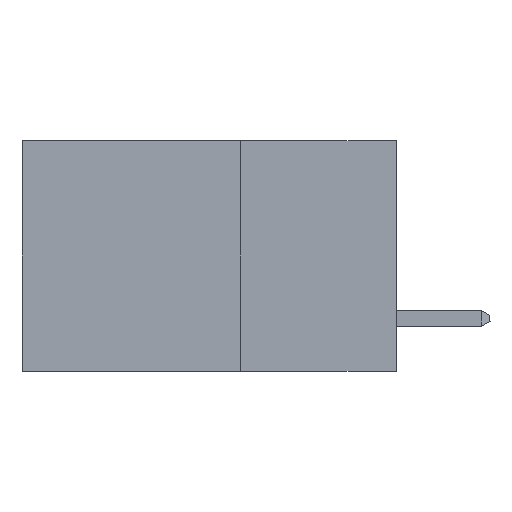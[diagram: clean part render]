
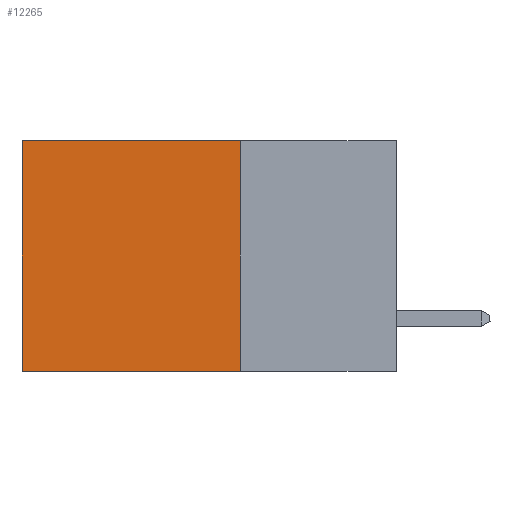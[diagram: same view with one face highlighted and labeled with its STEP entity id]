
A CAD part, left-side view. The second image highlights one B-rep face of the part: STEP entity #12265.
In plain terms, the highlighted planar face has unit normal (-1, 0, 0).
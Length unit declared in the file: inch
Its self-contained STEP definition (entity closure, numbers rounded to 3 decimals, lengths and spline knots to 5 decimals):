
#1314 = CARTESIAN_POINT ( 'NONE',  ( 0.298, 0.25, -0.37 ) ) ;
#1903 = VECTOR ( 'NONE', #5200, 39.37008 ) ;
#2294 = LINE ( 'NONE', #10504, #6072 ) ;
#2496 = VECTOR ( 'NONE', #14738, 39.37008 ) ;
#2888 = LINE ( 'NONE', #11260, #2496 ) ;
#3197 = ORIENTED_EDGE ( 'NONE', *, *, #7433, .F. ) ;
#3835 = DIRECTION ( 'NONE',  ( 1., 0., 0. ) ) ;
#4267 = ORIENTED_EDGE ( 'NONE', *, *, #6410, .T. ) ;
#5200 = DIRECTION ( 'NONE',  ( 0., 0., -1. ) ) ;
#5435 = CARTESIAN_POINT ( 'NONE',  ( 0.298, 0.6, 0. ) ) ;
#5701 = LINE ( 'NONE', #10752, #1903 ) ;
#6072 = VECTOR ( 'NONE', #12417, 39.37008 ) ;
#6164 = DIRECTION ( 'NONE',  ( 0., 1., 0. ) ) ;
#6410 = EDGE_CURVE ( 'NONE', #11763, #14839, #2294, .T. ) ;
#7433 = EDGE_CURVE ( 'NONE', #15279, #11608, #5701, .T. ) ;
#7614 = CARTESIAN_POINT ( 'NONE',  ( 0.298, 0.25, 0. ) ) ;
#9428 = CARTESIAN_POINT ( 'NONE',  ( 0.298, 0.25, 0. ) ) ;
#9562 = ORIENTED_EDGE ( 'NONE', *, *, #10904, .F. ) ;
#10504 = CARTESIAN_POINT ( 'NONE',  ( 0.298, 0.6, 0. ) ) ;
#10603 = LINE ( 'NONE', #12222, #13669 ) ;
#10654 = AXIS2_PLACEMENT_3D ( 'NONE', #7614, #3835, #12435 ) ;
#10752 = CARTESIAN_POINT ( 'NONE',  ( 0.298, 0.25, 0. ) ) ;
#10904 = EDGE_CURVE ( 'NONE', #11608, #14839, #10603, .T. ) ;
#11089 = ORIENTED_EDGE ( 'NONE', *, *, #12713, .T. ) ;
#11260 = CARTESIAN_POINT ( 'NONE',  ( 0.298, 0.25, 0. ) ) ;
#11272 = PLANE ( 'NONE',  #10654 ) ;
#11608 = VERTEX_POINT ( 'NONE', #1314 ) ;
#11763 = VERTEX_POINT ( 'NONE', #5435 ) ;
#12222 = CARTESIAN_POINT ( 'NONE',  ( 0.298, 0.25, -0.37 ) ) ;
#12265 = ADVANCED_FACE ( 'NONE', ( #13807 ), #11272, .F. ) ;
#12417 = DIRECTION ( 'NONE',  ( 0., 0., -1. ) ) ;
#12435 = DIRECTION ( 'NONE',  ( 0., 0., -1. ) ) ;
#12713 = EDGE_CURVE ( 'NONE', #15279, #11763, #2888, .T. ) ;
#13669 = VECTOR ( 'NONE', #6164, 39.37008 ) ;
#13807 = FACE_OUTER_BOUND ( 'NONE', #13974, .T. ) ;
#13974 = EDGE_LOOP ( 'NONE', ( #4267, #9562, #3197, #11089 ) ) ;
#14477 = CARTESIAN_POINT ( 'NONE',  ( 0.298, 0.6, -0.37 ) ) ;
#14738 = DIRECTION ( 'NONE',  ( 0., 1., 0. ) ) ;
#14839 = VERTEX_POINT ( 'NONE', #14477 ) ;
#15279 = VERTEX_POINT ( 'NONE', #9428 ) ;
